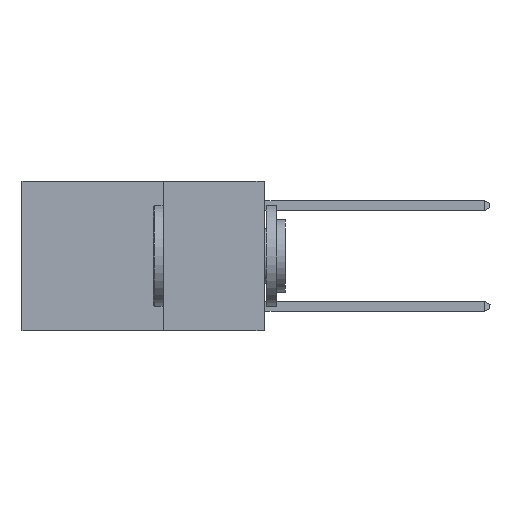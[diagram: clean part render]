
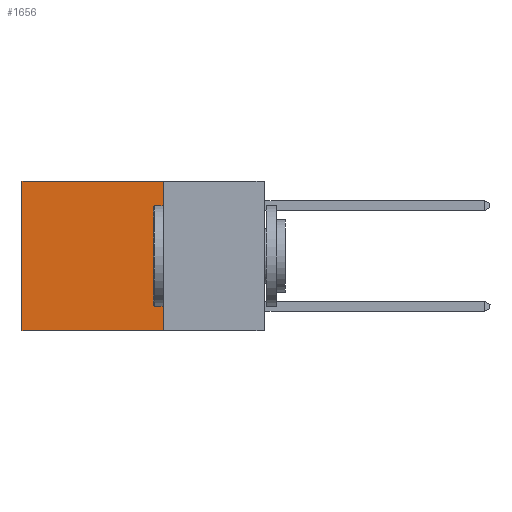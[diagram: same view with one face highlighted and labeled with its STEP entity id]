
A CAD part, left-side view. The second image highlights one B-rep face of the part: STEP entity #1656.
In plain terms, the highlighted planar face has unit normal (-1, 0, 0).
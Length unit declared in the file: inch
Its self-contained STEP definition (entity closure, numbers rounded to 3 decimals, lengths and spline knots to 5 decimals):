
#1656 = ADVANCED_FACE ( 'NONE', ( #18646 ), #23970, .F. ) ;
#1944 = CARTESIAN_POINT ( 'NONE',  ( 0.2625, 0.6, 0. ) ) ;
#3751 = ORIENTED_EDGE ( 'NONE', *, *, #4223, .F. ) ;
#4223 = EDGE_CURVE ( 'NONE', #17734, #10128, #13559, .T. ) ;
#4637 = ORIENTED_EDGE ( 'NONE', *, *, #9893, .T. ) ;
#6415 = CARTESIAN_POINT ( 'NONE',  ( 0.2625, 0.25, 0. ) ) ;
#6937 = CARTESIAN_POINT ( 'NONE',  ( 0.2625, 0.25, 0. ) ) ;
#7799 = AXIS2_PLACEMENT_3D ( 'NONE', #6937, #24077, #9414 ) ;
#8688 = DIRECTION ( 'NONE',  ( 0., 1., 0. ) ) ;
#8945 = DIRECTION ( 'NONE',  ( 0., 0., -1. ) ) ;
#9414 = DIRECTION ( 'NONE',  ( 0., 0., -1. ) ) ;
#9893 = EDGE_CURVE ( 'NONE', #16486, #17967, #29060, .T. ) ;
#10128 = VERTEX_POINT ( 'NONE', #29980 ) ;
#11414 = ORIENTED_EDGE ( 'NONE', *, *, #16397, .T. ) ;
#11469 = CARTESIAN_POINT ( 'NONE',  ( 0.2625, 0.6, -0.37 ) ) ;
#12230 = CARTESIAN_POINT ( 'NONE',  ( 0.2625, 0.6, 0. ) ) ;
#12688 = EDGE_LOOP ( 'NONE', ( #4637, #30684, #3751, #11414 ) ) ;
#12990 = CARTESIAN_POINT ( 'NONE',  ( 0.2625, 0.25, 0. ) ) ;
#13538 = CARTESIAN_POINT ( 'NONE',  ( 0.2625, 0.25, -0.37 ) ) ;
#13559 = LINE ( 'NONE', #13802, #25742 ) ;
#13802 = CARTESIAN_POINT ( 'NONE',  ( 0.2625, 0.25, 0. ) ) ;
#15714 = VECTOR ( 'NONE', #26094, 39.37008 ) ;
#16289 = EDGE_CURVE ( 'NONE', #10128, #17967, #18817, .T. ) ;
#16397 = EDGE_CURVE ( 'NONE', #17734, #16486, #16489, .T. ) ;
#16486 = VERTEX_POINT ( 'NONE', #1944 ) ;
#16489 = LINE ( 'NONE', #6415, #15714 ) ;
#17734 = VERTEX_POINT ( 'NONE', #12990 ) ;
#17967 = VERTEX_POINT ( 'NONE', #11469 ) ;
#18646 = FACE_OUTER_BOUND ( 'NONE', #12688, .T. ) ;
#18817 = LINE ( 'NONE', #13538, #24526 ) ;
#23970 = PLANE ( 'NONE',  #7799 ) ;
#24077 = DIRECTION ( 'NONE',  ( 1., 0., 0. ) ) ;
#24526 = VECTOR ( 'NONE', #8688, 39.37008 ) ;
#25742 = VECTOR ( 'NONE', #8945, 39.37008 ) ;
#26094 = DIRECTION ( 'NONE',  ( 0., 1., 0. ) ) ;
#26925 = DIRECTION ( 'NONE',  ( 0., 0., -1. ) ) ;
#29060 = LINE ( 'NONE', #12230, #30562 ) ;
#29980 = CARTESIAN_POINT ( 'NONE',  ( 0.2625, 0.25, -0.37 ) ) ;
#30562 = VECTOR ( 'NONE', #26925, 39.37008 ) ;
#30684 = ORIENTED_EDGE ( 'NONE', *, *, #16289, .F. ) ;
